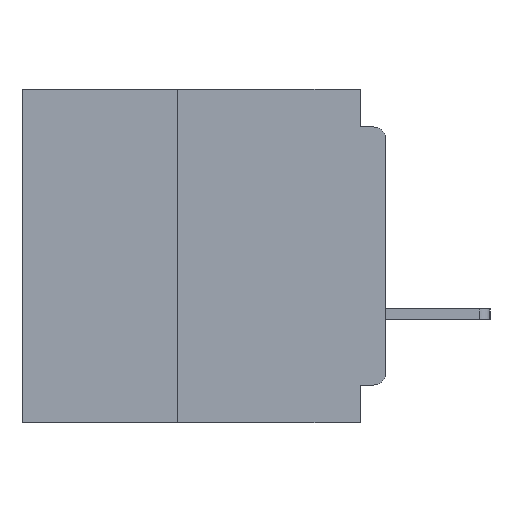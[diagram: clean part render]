
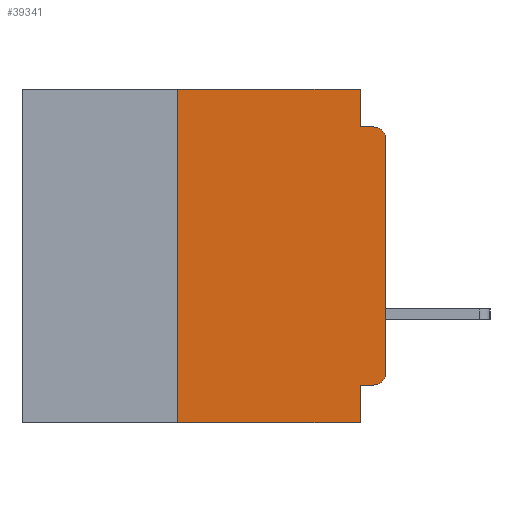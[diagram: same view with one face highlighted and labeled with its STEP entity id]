
A CAD part, left-side view. The second image highlights one B-rep face of the part: STEP entity #39341.
In plain terms, the highlighted planar face has unit normal (-1, 0, 0).
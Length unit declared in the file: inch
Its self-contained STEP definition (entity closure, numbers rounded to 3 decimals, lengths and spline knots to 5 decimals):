
#118 = DIRECTION ( 'NONE',  ( 0., -1., 0. ) ) ;
#721 = ORIENTED_EDGE ( 'NONE', *, *, #53053, .F. ) ;
#3468 = LINE ( 'NONE', #15060, #54830 ) ;
#4285 = LINE ( 'NONE', #10548, #14519 ) ;
#5334 = LINE ( 'NONE', #31636, #30484 ) ;
#5627 = VERTEX_POINT ( 'NONE', #64179 ) ;
#5893 = DIRECTION ( 'NONE',  ( 0., 0., 1. ) ) ;
#6098 = VERTEX_POINT ( 'NONE', #58748 ) ;
#6663 = AXIS2_PLACEMENT_3D ( 'NONE', #24722, #59406, #29821 ) ;
#7471 = VECTOR ( 'NONE', #42483, 39.37008 ) ;
#7607 = CARTESIAN_POINT ( 'NONE',  ( 0., 0., 0. ) ) ;
#8815 = EDGE_CURVE ( 'NONE', #35194, #25026, #10326, .T. ) ;
#9130 = VERTEX_POINT ( 'NONE', #11479 ) ;
#9381 = ORIENTED_EDGE ( 'NONE', *, *, #8815, .F. ) ;
#10119 = LINE ( 'NONE', #59816, #48229 ) ;
#10326 = LINE ( 'NONE', #58646, #61610 ) ;
#10548 = CARTESIAN_POINT ( 'NONE',  ( 0., 0.25, -0.4 ) ) ;
#10608 = ORIENTED_EDGE ( 'NONE', *, *, #34542, .T. ) ;
#11076 = ORIENTED_EDGE ( 'NONE', *, *, #32206, .F. ) ;
#11479 = CARTESIAN_POINT ( 'NONE',  ( 0., 0.031, -0.045 ) ) ;
#13577 = CARTESIAN_POINT ( 'NONE',  ( 0., 0.015, -0.355 ) ) ;
#14351 = CARTESIAN_POINT ( 'NONE',  ( 0., 0.031, -0.355 ) ) ;
#14519 = VECTOR ( 'NONE', #5893, 39.37008 ) ;
#14741 = PLANE ( 'NONE',  #6663 ) ;
#15060 = CARTESIAN_POINT ( 'NONE',  ( 0., 0.437, -0.4 ) ) ;
#15845 = VERTEX_POINT ( 'NONE', #40905 ) ;
#17107 = FACE_OUTER_BOUND ( 'NONE', #47906, .T. ) ;
#17278 = VERTEX_POINT ( 'NONE', #27983 ) ;
#17607 = CARTESIAN_POINT ( 'NONE',  ( 0., 0.015, -0.06 ) ) ;
#18840 = CIRCLE ( 'NONE', #35511, 0.015 ) ;
#22573 = CARTESIAN_POINT ( 'NONE',  ( 0., 0.015, -0.34 ) ) ;
#22621 = DIRECTION ( 'NONE',  ( 0., 0., -1. ) ) ;
#23757 = EDGE_CURVE ( 'NONE', #62974, #17278, #58835, .T. ) ;
#23972 = DIRECTION ( 'NONE',  ( 0., 0., -1. ) ) ;
#24722 = CARTESIAN_POINT ( 'NONE',  ( 0., 0.437, 0. ) ) ;
#25026 = VERTEX_POINT ( 'NONE', #52458 ) ;
#26313 = DIRECTION ( 'NONE',  ( 0., 0., -1. ) ) ;
#26702 = AXIS2_PLACEMENT_3D ( 'NONE', #17607, #52272, #22621 ) ;
#27600 = DIRECTION ( 'NONE',  ( 0., 0., -1. ) ) ;
#27983 = CARTESIAN_POINT ( 'NONE',  ( 0., 0., -0.06 ) ) ;
#28501 = CARTESIAN_POINT ( 'NONE',  ( 0., 0., -0.045 ) ) ;
#29821 = DIRECTION ( 'NONE',  ( 0., 0., -1. ) ) ;
#30484 = VECTOR ( 'NONE', #36564, 39.37008 ) ;
#30499 = EDGE_CURVE ( 'NONE', #17278, #5627, #60085, .T. ) ;
#31636 = CARTESIAN_POINT ( 'NONE',  ( 0., 0.437, 0. ) ) ;
#32206 = EDGE_CURVE ( 'NONE', #36274, #35194, #10119, .T. ) ;
#33422 = VECTOR ( 'NONE', #33521, 39.37008 ) ;
#33521 = DIRECTION ( 'NONE',  ( 0., -1., 0. ) ) ;
#34542 = EDGE_CURVE ( 'NONE', #47316, #25026, #3468, .T. ) ;
#35113 = LINE ( 'NONE', #56002, #58313 ) ;
#35194 = VERTEX_POINT ( 'NONE', #14351 ) ;
#35511 = AXIS2_PLACEMENT_3D ( 'NONE', #22573, #57251, #27600 ) ;
#36274 = VERTEX_POINT ( 'NONE', #13577 ) ;
#36564 = DIRECTION ( 'NONE',  ( 0., -1., 0. ) ) ;
#36684 = ORIENTED_EDGE ( 'NONE', *, *, #37437, .T. ) ;
#36686 = CARTESIAN_POINT ( 'NONE',  ( 0., 0., -0.34 ) ) ;
#37437 = EDGE_CURVE ( 'NONE', #36274, #62974, #18840, .T. ) ;
#38093 = ORIENTED_EDGE ( 'NONE', *, *, #62358, .F. ) ;
#38933 = EDGE_CURVE ( 'NONE', #15845, #9130, #35113, .T. ) ;
#38956 = EDGE_CURVE ( 'NONE', #6098, #15845, #5334, .T. ) ;
#39341 = ADVANCED_FACE ( 'NONE', ( #17107 ), #14741, .F. ) ;
#40905 = CARTESIAN_POINT ( 'NONE',  ( 0., 0.031, 0. ) ) ;
#42483 = DIRECTION ( 'NONE',  ( 0., 0., 1. ) ) ;
#45997 = ORIENTED_EDGE ( 'NONE', *, *, #38956, .F. ) ;
#47316 = VERTEX_POINT ( 'NONE', #60563 ) ;
#47906 = EDGE_LOOP ( 'NONE', ( #60662, #58809, #721, #56751, #45997, #38093, #10608, #9381, #11076, #36684 ) ) ;
#48229 = VECTOR ( 'NONE', #50052, 39.37008 ) ;
#50052 = DIRECTION ( 'NONE',  ( 0., 1., 0. ) ) ;
#52272 = DIRECTION ( 'NONE',  ( -1., 0., 0. ) ) ;
#52458 = CARTESIAN_POINT ( 'NONE',  ( 0., 0.031, -0.4 ) ) ;
#53053 = EDGE_CURVE ( 'NONE', #9130, #5627, #59675, .T. ) ;
#54830 = VECTOR ( 'NONE', #118, 39.37008 ) ;
#56002 = CARTESIAN_POINT ( 'NONE',  ( 0., 0.031, 0. ) ) ;
#56751 = ORIENTED_EDGE ( 'NONE', *, *, #38933, .F. ) ;
#57251 = DIRECTION ( 'NONE',  ( -1., 0., 0. ) ) ;
#58313 = VECTOR ( 'NONE', #26313, 39.37008 ) ;
#58646 = CARTESIAN_POINT ( 'NONE',  ( 0., 0.031, -0.4 ) ) ;
#58748 = CARTESIAN_POINT ( 'NONE',  ( 0., 0.25, 0. ) ) ;
#58809 = ORIENTED_EDGE ( 'NONE', *, *, #30499, .T. ) ;
#58835 = LINE ( 'NONE', #7607, #7471 ) ;
#59406 = DIRECTION ( 'NONE',  ( 1., 0., 0. ) ) ;
#59675 = LINE ( 'NONE', #28501, #33422 ) ;
#59816 = CARTESIAN_POINT ( 'NONE',  ( 0., 0., -0.355 ) ) ;
#60085 = CIRCLE ( 'NONE', #26702, 0.015 ) ;
#60563 = CARTESIAN_POINT ( 'NONE',  ( 0., 0.25, -0.4 ) ) ;
#60662 = ORIENTED_EDGE ( 'NONE', *, *, #23757, .T. ) ;
#61610 = VECTOR ( 'NONE', #23972, 39.37008 ) ;
#62358 = EDGE_CURVE ( 'NONE', #47316, #6098, #4285, .T. ) ;
#62974 = VERTEX_POINT ( 'NONE', #36686 ) ;
#64179 = CARTESIAN_POINT ( 'NONE',  ( 0., 0.015, -0.045 ) ) ;
